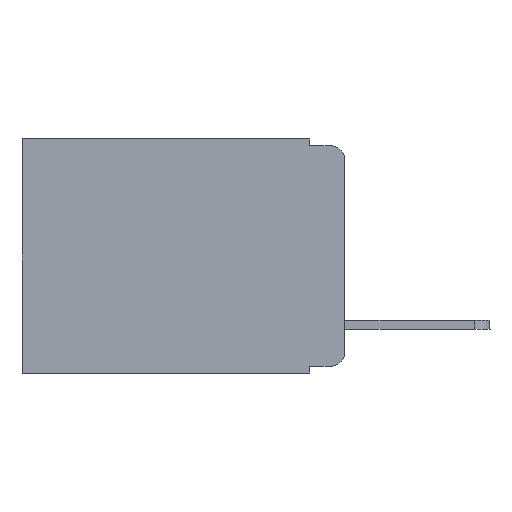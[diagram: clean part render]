
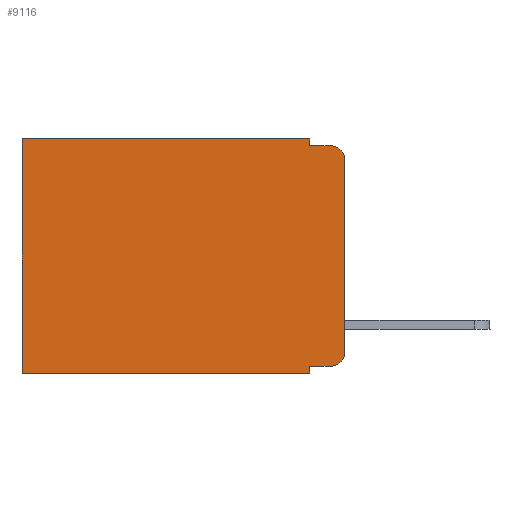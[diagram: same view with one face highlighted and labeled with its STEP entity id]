
A CAD part, left-side view. The second image highlights one B-rep face of the part: STEP entity #9116.
In plain terms, the highlighted planar face has unit normal (-1, 0, 0).
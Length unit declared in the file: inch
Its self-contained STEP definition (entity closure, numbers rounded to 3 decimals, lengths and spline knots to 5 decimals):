
#230 = CARTESIAN_POINT ( 'NONE',  ( 0.298, 0.051, -0.01 ) ) ;
#399 = VECTOR ( 'NONE', #1206, 39.37008 ) ;
#633 = DIRECTION ( 'NONE',  ( 0., 0., -1. ) ) ;
#865 = CARTESIAN_POINT ( 'NONE',  ( 0.298, 0., -0.343 ) ) ;
#937 = EDGE_CURVE ( 'NONE', #13358, #9528, #2223, .T. ) ;
#974 = DIRECTION ( 'NONE',  ( 0., 0., -1. ) ) ;
#1206 = DIRECTION ( 'NONE',  ( 0., -1., 0. ) ) ;
#1339 = EDGE_CURVE ( 'NONE', #7672, #10857, #4191, .T. ) ;
#1366 = DIRECTION ( 'NONE',  ( 0., -1., 0. ) ) ;
#1545 = EDGE_CURVE ( 'NONE', #11070, #9074, #9614, .T. ) ;
#1562 = DIRECTION ( 'NONE',  ( -1., 0., 0. ) ) ;
#1809 = CARTESIAN_POINT ( 'NONE',  ( 0.298, 0.051, 0. ) ) ;
#1851 = CARTESIAN_POINT ( 'NONE',  ( 0.298, 0.051, -0.01 ) ) ;
#1885 = CARTESIAN_POINT ( 'NONE',  ( 0.298, 0., -0.313 ) ) ;
#1895 = ORIENTED_EDGE ( 'NONE', *, *, #3599, .F. ) ;
#2223 = LINE ( 'NONE', #6564, #12933 ) ;
#2248 = CARTESIAN_POINT ( 'NONE',  ( 0.298, 0.051, -0.333 ) ) ;
#2521 = VERTEX_POINT ( 'NONE', #7815 ) ;
#2782 = CARTESIAN_POINT ( 'NONE',  ( 0.298, 0., 0. ) ) ;
#2960 = CARTESIAN_POINT ( 'NONE',  ( 0.298, 0.473, -0.343 ) ) ;
#3111 = VERTEX_POINT ( 'NONE', #1851 ) ;
#3280 = CIRCLE ( 'NONE', #13224, 0.02 ) ;
#3456 = CARTESIAN_POINT ( 'NONE',  ( 0.298, 0.051, 0. ) ) ;
#3494 = EDGE_CURVE ( 'NONE', #10284, #3111, #13369, .T. ) ;
#3504 = VERTEX_POINT ( 'NONE', #1885 ) ;
#3509 = VECTOR ( 'NONE', #13589, 39.37008 ) ;
#3599 = EDGE_CURVE ( 'NONE', #3111, #9074, #5479, .T. ) ;
#3703 = CARTESIAN_POINT ( 'NONE',  ( 0.298, 0.473, 0. ) ) ;
#3762 = VECTOR ( 'NONE', #12506, 39.37008 ) ;
#3832 = DIRECTION ( 'NONE',  ( 0., 0., -1. ) ) ;
#3900 = LINE ( 'NONE', #7006, #6603 ) ;
#4191 = LINE ( 'NONE', #2248, #8930 ) ;
#4561 = CARTESIAN_POINT ( 'NONE',  ( 0.298, 0., -0.03 ) ) ;
#4932 = AXIS2_PLACEMENT_3D ( 'NONE', #6788, #1562, #3832 ) ;
#5015 = DIRECTION ( 'NONE',  ( -1., 0., 0. ) ) ;
#5033 = CARTESIAN_POINT ( 'NONE',  ( 0.298, 0., 0. ) ) ;
#5232 = ORIENTED_EDGE ( 'NONE', *, *, #3494, .F. ) ;
#5238 = ORIENTED_EDGE ( 'NONE', *, *, #1545, .T. ) ;
#5356 = DIRECTION ( 'NONE',  ( 0., 1., 0. ) ) ;
#5479 = LINE ( 'NONE', #230, #399 ) ;
#6042 = ORIENTED_EDGE ( 'NONE', *, *, #11607, .T. ) ;
#6240 = LINE ( 'NONE', #865, #3762 ) ;
#6564 = CARTESIAN_POINT ( 'NONE',  ( 0.298, 0.473, 0. ) ) ;
#6603 = VECTOR ( 'NONE', #11259, 39.37008 ) ;
#6788 = CARTESIAN_POINT ( 'NONE',  ( 0.298, 0.02, -0.03 ) ) ;
#7006 = CARTESIAN_POINT ( 'NONE',  ( 0.298, 0.051, 0. ) ) ;
#7120 = LINE ( 'NONE', #2782, #12570 ) ;
#7160 = DIRECTION ( 'NONE',  ( 0., 0., -1. ) ) ;
#7251 = PLANE ( 'NONE',  #11672 ) ;
#7672 = VERTEX_POINT ( 'NONE', #10111 ) ;
#7775 = LINE ( 'NONE', #9674, #13068 ) ;
#7815 = CARTESIAN_POINT ( 'NONE',  ( 0.298, 0.051, -0.343 ) ) ;
#8930 = VECTOR ( 'NONE', #1366, 39.37008 ) ;
#8992 = CARTESIAN_POINT ( 'NONE',  ( 0.298, 0.02, -0.333 ) ) ;
#9074 = VERTEX_POINT ( 'NONE', #13488 ) ;
#9116 = ADVANCED_FACE ( 'NONE', ( #10323 ), #7251, .F. ) ;
#9256 = CARTESIAN_POINT ( 'NONE',  ( 0.298, 0.02, -0.313 ) ) ;
#9479 = EDGE_CURVE ( 'NONE', #10857, #3504, #3280, .T. ) ;
#9512 = ORIENTED_EDGE ( 'NONE', *, *, #10473, .F. ) ;
#9528 = VERTEX_POINT ( 'NONE', #2960 ) ;
#9562 = ORIENTED_EDGE ( 'NONE', *, *, #9479, .T. ) ;
#9614 = CIRCLE ( 'NONE', #4932, 0.02 ) ;
#9674 = CARTESIAN_POINT ( 'NONE',  ( 0.298, 0., 0. ) ) ;
#10111 = CARTESIAN_POINT ( 'NONE',  ( 0.298, 0.051, -0.333 ) ) ;
#10284 = VERTEX_POINT ( 'NONE', #3456 ) ;
#10323 = FACE_OUTER_BOUND ( 'NONE', #10470, .T. ) ;
#10470 = EDGE_LOOP ( 'NONE', ( #9512, #5238, #1895, #5232, #6042, #13445, #12399, #12577, #12382, #9562 ) ) ;
#10473 = EDGE_CURVE ( 'NONE', #11070, #3504, #7120, .T. ) ;
#10857 = VERTEX_POINT ( 'NONE', #8992 ) ;
#11070 = VERTEX_POINT ( 'NONE', #4561 ) ;
#11259 = DIRECTION ( 'NONE',  ( 0., 0., -1. ) ) ;
#11507 = DIRECTION ( 'NONE',  ( 1., 0., 0. ) ) ;
#11607 = EDGE_CURVE ( 'NONE', #10284, #13358, #7775, .T. ) ;
#11672 = AXIS2_PLACEMENT_3D ( 'NONE', #5033, #11507, #974 ) ;
#11791 = EDGE_CURVE ( 'NONE', #7672, #2521, #3900, .T. ) ;
#11819 = EDGE_CURVE ( 'NONE', #2521, #9528, #6240, .T. ) ;
#12382 = ORIENTED_EDGE ( 'NONE', *, *, #1339, .T. ) ;
#12399 = ORIENTED_EDGE ( 'NONE', *, *, #11819, .F. ) ;
#12506 = DIRECTION ( 'NONE',  ( 0., 1., 0. ) ) ;
#12570 = VECTOR ( 'NONE', #633, 39.37008 ) ;
#12577 = ORIENTED_EDGE ( 'NONE', *, *, #11791, .F. ) ;
#12699 = DIRECTION ( 'NONE',  ( 0., 0., -1. ) ) ;
#12933 = VECTOR ( 'NONE', #12699, 39.37008 ) ;
#13068 = VECTOR ( 'NONE', #5356, 39.37008 ) ;
#13224 = AXIS2_PLACEMENT_3D ( 'NONE', #9256, #5015, #7160 ) ;
#13358 = VERTEX_POINT ( 'NONE', #3703 ) ;
#13369 = LINE ( 'NONE', #1809, #3509 ) ;
#13445 = ORIENTED_EDGE ( 'NONE', *, *, #937, .T. ) ;
#13488 = CARTESIAN_POINT ( 'NONE',  ( 0.298, 0.02, -0.01 ) ) ;
#13589 = DIRECTION ( 'NONE',  ( 0., 0., -1. ) ) ;
